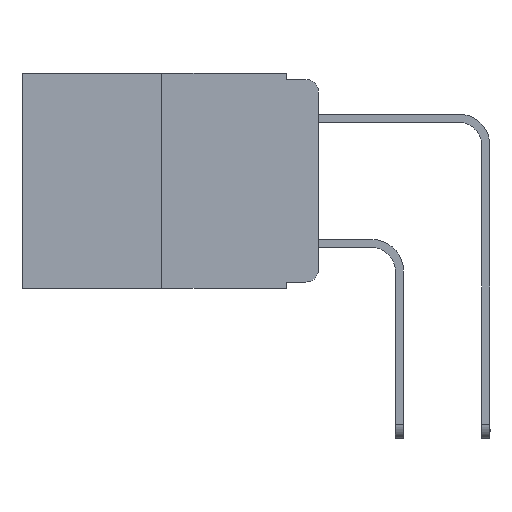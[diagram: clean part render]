
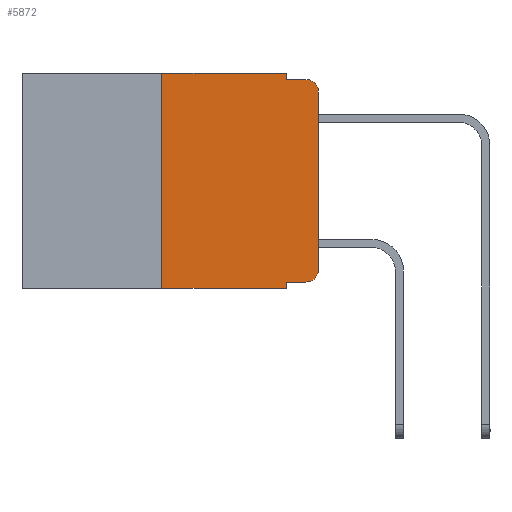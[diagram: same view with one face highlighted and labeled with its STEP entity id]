
A CAD part, left-side view. The second image highlights one B-rep face of the part: STEP entity #5872.
In plain terms, the highlighted planar face has unit normal (-1, 0, 0).
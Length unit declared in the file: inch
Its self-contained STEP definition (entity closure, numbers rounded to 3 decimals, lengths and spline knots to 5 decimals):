
#128 = ORIENTED_EDGE ( 'NONE', *, *, #11968, .F. ) ;
#278 = VECTOR ( 'NONE', #3661, 39.37008 ) ;
#284 = CARTESIAN_POINT ( 'NONE',  ( 0., 0.25, -0.343 ) ) ;
#402 = VERTEX_POINT ( 'NONE', #13028 ) ;
#708 = CARTESIAN_POINT ( 'NONE',  ( 0., 0.051, 0. ) ) ;
#925 = CARTESIAN_POINT ( 'NONE',  ( 0., 0.25, 0. ) ) ;
#930 = EDGE_CURVE ( 'NONE', #2770, #9579, #11456, .T. ) ;
#1269 = EDGE_CURVE ( 'NONE', #12089, #6042, #9932, .T. ) ;
#1465 = VECTOR ( 'NONE', #5512, 39.37008 ) ;
#1546 = CARTESIAN_POINT ( 'NONE',  ( 0., 0.473, -0.343 ) ) ;
#1737 = CIRCLE ( 'NONE', #10703, 0.02 ) ;
#1903 = DIRECTION ( 'NONE',  ( 0., 0., -1. ) ) ;
#1970 = DIRECTION ( 'NONE',  ( -1., 0., 0. ) ) ;
#1972 = VECTOR ( 'NONE', #2957, 39.37008 ) ;
#2005 = DIRECTION ( 'NONE',  ( -1., 0., 0. ) ) ;
#2268 = CARTESIAN_POINT ( 'NONE',  ( 0., 0.051, 0. ) ) ;
#2512 = DIRECTION ( 'NONE',  ( 0., -1., 0. ) ) ;
#2686 = EDGE_LOOP ( 'NONE', ( #7819, #4719, #8968, #11929, #12861, #128, #10769, #7702, #10423, #4579 ) ) ;
#2702 = DIRECTION ( 'NONE',  ( 0., -1., 0. ) ) ;
#2770 = VERTEX_POINT ( 'NONE', #10245 ) ;
#2957 = DIRECTION ( 'NONE',  ( 0., 0., -1. ) ) ;
#3021 = CARTESIAN_POINT ( 'NONE',  ( 0., 0.02, -0.03 ) ) ;
#3661 = DIRECTION ( 'NONE',  ( 0., 0., 1. ) ) ;
#3799 = VERTEX_POINT ( 'NONE', #13829 ) ;
#4044 = DIRECTION ( 'NONE',  ( 0., 0., -1. ) ) ;
#4094 = CARTESIAN_POINT ( 'NONE',  ( 0., 0.02, -0.313 ) ) ;
#4221 = LINE ( 'NONE', #1546, #6056 ) ;
#4305 = EDGE_CURVE ( 'NONE', #11709, #3799, #11569, .T. ) ;
#4325 = CARTESIAN_POINT ( 'NONE',  ( 0., 0.051, -0.333 ) ) ;
#4579 = ORIENTED_EDGE ( 'NONE', *, *, #7521, .T. ) ;
#4676 = VECTOR ( 'NONE', #7693, 39.37008 ) ;
#4719 = ORIENTED_EDGE ( 'NONE', *, *, #4305, .T. ) ;
#5351 = AXIS2_PLACEMENT_3D ( 'NONE', #3021, #2005, #1903 ) ;
#5490 = VECTOR ( 'NONE', #2702, 39.37008 ) ;
#5512 = DIRECTION ( 'NONE',  ( 0., 0., -1. ) ) ;
#5691 = DIRECTION ( 'NONE',  ( 0., 0., -1. ) ) ;
#5774 = CARTESIAN_POINT ( 'NONE',  ( 0., 0., 0. ) ) ;
#5872 = ADVANCED_FACE ( 'NONE', ( #10678 ), #7969, .F. ) ;
#5929 = CARTESIAN_POINT ( 'NONE',  ( 0., 0.02, -0.333 ) ) ;
#6042 = VERTEX_POINT ( 'NONE', #10376 ) ;
#6056 = VECTOR ( 'NONE', #13423, 39.37008 ) ;
#7088 = VERTEX_POINT ( 'NONE', #284 ) ;
#7407 = VECTOR ( 'NONE', #13796, 39.37008 ) ;
#7521 = EDGE_CURVE ( 'NONE', #13085, #11899, #1737, .T. ) ;
#7591 = EDGE_CURVE ( 'NONE', #12089, #13085, #13044, .T. ) ;
#7693 = DIRECTION ( 'NONE',  ( 0., -1., 0. ) ) ;
#7702 = ORIENTED_EDGE ( 'NONE', *, *, #1269, .F. ) ;
#7819 = ORIENTED_EDGE ( 'NONE', *, *, #12297, .T. ) ;
#7969 = PLANE ( 'NONE',  #12546 ) ;
#8009 = DIRECTION ( 'NONE',  ( 1., 0., 0. ) ) ;
#8489 = CARTESIAN_POINT ( 'NONE',  ( 0., 0., -0.313 ) ) ;
#8777 = CARTESIAN_POINT ( 'NONE',  ( 0., 0.051, -0.01 ) ) ;
#8929 = LINE ( 'NONE', #925, #7407 ) ;
#8968 = ORIENTED_EDGE ( 'NONE', *, *, #13741, .F. ) ;
#9029 = EDGE_CURVE ( 'NONE', #402, #2770, #13160, .T. ) ;
#9576 = LINE ( 'NONE', #5774, #278 ) ;
#9579 = VERTEX_POINT ( 'NONE', #8777 ) ;
#9932 = LINE ( 'NONE', #708, #1972 ) ;
#10067 = CARTESIAN_POINT ( 'NONE',  ( 0., 0.473, 0. ) ) ;
#10229 = CARTESIAN_POINT ( 'NONE',  ( 0., 0.051, -0.01 ) ) ;
#10245 = CARTESIAN_POINT ( 'NONE',  ( 0., 0.051, 0. ) ) ;
#10376 = CARTESIAN_POINT ( 'NONE',  ( 0., 0.051, -0.343 ) ) ;
#10423 = ORIENTED_EDGE ( 'NONE', *, *, #7591, .T. ) ;
#10676 = CARTESIAN_POINT ( 'NONE',  ( 0., 0.051, -0.333 ) ) ;
#10678 = FACE_OUTER_BOUND ( 'NONE', #2686, .T. ) ;
#10703 = AXIS2_PLACEMENT_3D ( 'NONE', #4094, #1970, #4044 ) ;
#10769 = ORIENTED_EDGE ( 'NONE', *, *, #11161, .T. ) ;
#11161 = EDGE_CURVE ( 'NONE', #7088, #6042, #4221, .T. ) ;
#11337 = VECTOR ( 'NONE', #2512, 39.37008 ) ;
#11456 = LINE ( 'NONE', #2268, #1465 ) ;
#11569 = CIRCLE ( 'NONE', #5351, 0.02 ) ;
#11709 = VERTEX_POINT ( 'NONE', #12176 ) ;
#11899 = VERTEX_POINT ( 'NONE', #8489 ) ;
#11929 = ORIENTED_EDGE ( 'NONE', *, *, #930, .F. ) ;
#11968 = EDGE_CURVE ( 'NONE', #7088, #402, #8929, .T. ) ;
#12089 = VERTEX_POINT ( 'NONE', #4325 ) ;
#12176 = CARTESIAN_POINT ( 'NONE',  ( 0., 0., -0.03 ) ) ;
#12297 = EDGE_CURVE ( 'NONE', #11899, #11709, #9576, .T. ) ;
#12546 = AXIS2_PLACEMENT_3D ( 'NONE', #13358, #8009, #5691 ) ;
#12861 = ORIENTED_EDGE ( 'NONE', *, *, #9029, .F. ) ;
#13028 = CARTESIAN_POINT ( 'NONE',  ( 0., 0.25, 0. ) ) ;
#13044 = LINE ( 'NONE', #10676, #4676 ) ;
#13085 = VERTEX_POINT ( 'NONE', #5929 ) ;
#13160 = LINE ( 'NONE', #10067, #11337 ) ;
#13205 = LINE ( 'NONE', #10229, #5490 ) ;
#13358 = CARTESIAN_POINT ( 'NONE',  ( 0., 0.473, 0. ) ) ;
#13423 = DIRECTION ( 'NONE',  ( 0., -1., 0. ) ) ;
#13741 = EDGE_CURVE ( 'NONE', #9579, #3799, #13205, .T. ) ;
#13796 = DIRECTION ( 'NONE',  ( 0., 0., 1. ) ) ;
#13829 = CARTESIAN_POINT ( 'NONE',  ( 0., 0.02, -0.01 ) ) ;
